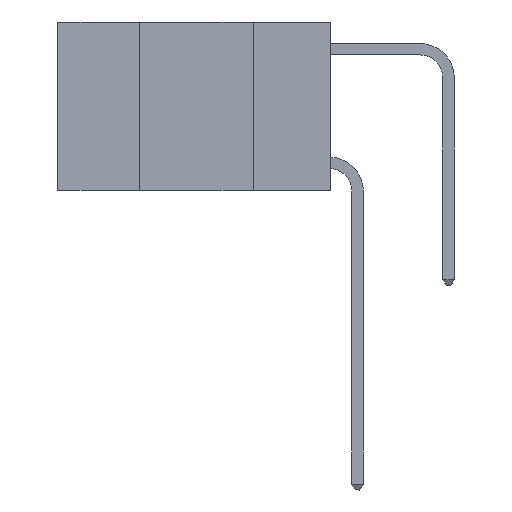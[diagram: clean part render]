
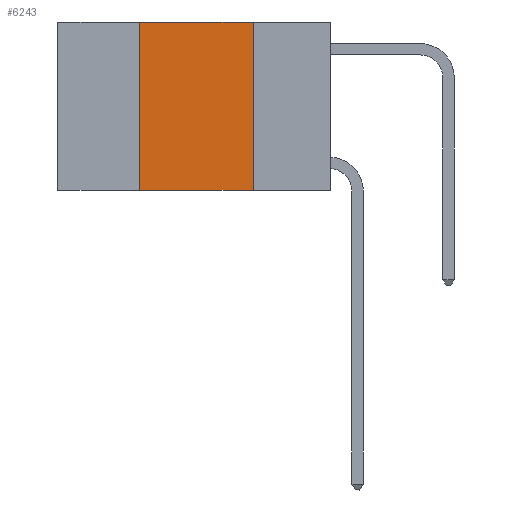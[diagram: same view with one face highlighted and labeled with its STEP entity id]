
A CAD part, left-side view. The second image highlights one B-rep face of the part: STEP entity #6243.
In plain terms, the highlighted planar face has unit normal (-1, 0, 0).
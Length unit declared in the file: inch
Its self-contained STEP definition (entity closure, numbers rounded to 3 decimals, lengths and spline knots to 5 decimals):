
#1820 = DIRECTION ( 'NONE',  ( 0., -1., 0. ) ) ;
#4352 = VERTEX_POINT ( 'NONE', #5429 ) ;
#5429 = CARTESIAN_POINT ( 'NONE',  ( 0., 0.17, 0. ) ) ;
#5543 = CARTESIAN_POINT ( 'NONE',  ( 0., 0.6, 0. ) ) ;
#6243 = ADVANCED_FACE ( 'NONE', ( #22671 ), #24760, .F. ) ;
#6381 = VECTOR ( 'NONE', #26521, 39.37008 ) ;
#7313 = CARTESIAN_POINT ( 'NONE',  ( 0., 0.42, -0.37 ) ) ;
#7445 = CARTESIAN_POINT ( 'NONE',  ( 0., 0.17, 0. ) ) ;
#7529 = ORIENTED_EDGE ( 'NONE', *, *, #22277, .F. ) ;
#7835 = EDGE_CURVE ( 'NONE', #14735, #15559, #17497, .T. ) ;
#8119 = CARTESIAN_POINT ( 'NONE',  ( 0., 0.42, 0. ) ) ;
#9715 = LINE ( 'NONE', #22786, #12825 ) ;
#11169 = CARTESIAN_POINT ( 'NONE',  ( 0., 0.42, 0. ) ) ;
#11497 = ORIENTED_EDGE ( 'NONE', *, *, #21527, .T. ) ;
#12398 = CARTESIAN_POINT ( 'NONE',  ( 0., 0.17, -0.37 ) ) ;
#12825 = VECTOR ( 'NONE', #26685, 39.37008 ) ;
#14108 = DIRECTION ( 'NONE',  ( 0., 0., -1. ) ) ;
#14735 = VERTEX_POINT ( 'NONE', #7313 ) ;
#15559 = VERTEX_POINT ( 'NONE', #8119 ) ;
#15756 = VERTEX_POINT ( 'NONE', #12398 ) ;
#15939 = EDGE_CURVE ( 'NONE', #4352, #15756, #17990, .T. ) ;
#16077 = ORIENTED_EDGE ( 'NONE', *, *, #15939, .F. ) ;
#17497 = LINE ( 'NONE', #11169, #22118 ) ;
#17703 = ORIENTED_EDGE ( 'NONE', *, *, #7835, .F. ) ;
#17990 = LINE ( 'NONE', #7445, #6381 ) ;
#19125 = VECTOR ( 'NONE', #1820, 39.37008 ) ;
#20775 = CARTESIAN_POINT ( 'NONE',  ( 0., 0.6, -0.37 ) ) ;
#21527 = EDGE_CURVE ( 'NONE', #14735, #15756, #27073, .T. ) ;
#22118 = VECTOR ( 'NONE', #24083, 39.37008 ) ;
#22277 = EDGE_CURVE ( 'NONE', #15559, #4352, #9715, .T. ) ;
#22671 = FACE_OUTER_BOUND ( 'NONE', #23147, .T. ) ;
#22786 = CARTESIAN_POINT ( 'NONE',  ( 0., 0.6, 0. ) ) ;
#22804 = DIRECTION ( 'NONE',  ( 1., 0., 0. ) ) ;
#23147 = EDGE_LOOP ( 'NONE', ( #16077, #7529, #17703, #11497 ) ) ;
#24083 = DIRECTION ( 'NONE',  ( 0., 0., 1. ) ) ;
#24760 = PLANE ( 'NONE',  #27387 ) ;
#26521 = DIRECTION ( 'NONE',  ( 0., 0., -1. ) ) ;
#26685 = DIRECTION ( 'NONE',  ( 0., -1., 0. ) ) ;
#27073 = LINE ( 'NONE', #20775, #19125 ) ;
#27387 = AXIS2_PLACEMENT_3D ( 'NONE', #5543, #22804, #14108 ) ;
